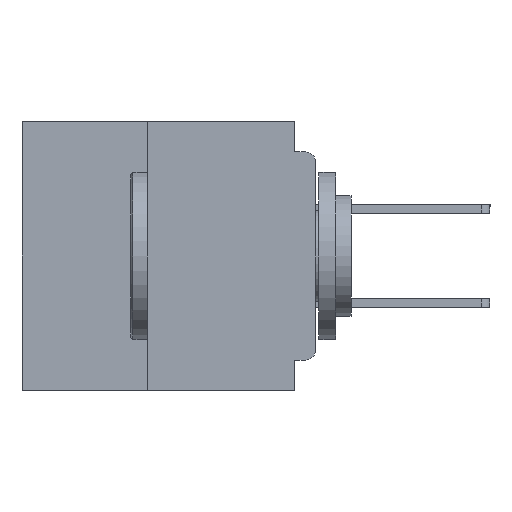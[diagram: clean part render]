
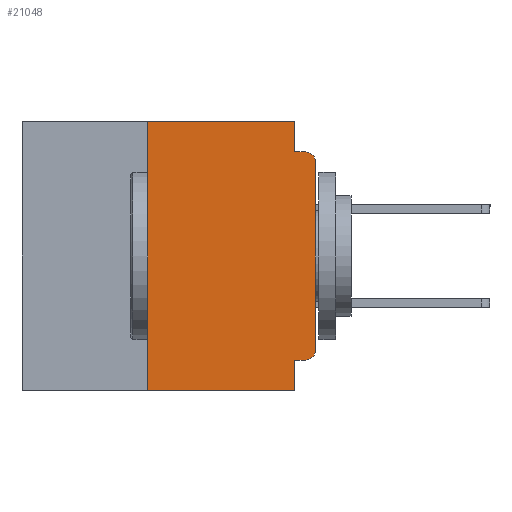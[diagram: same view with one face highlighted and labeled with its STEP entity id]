
A CAD part, left-side view. The second image highlights one B-rep face of the part: STEP entity #21048.
In plain terms, the highlighted planar face has unit normal (-1, 0, 0).
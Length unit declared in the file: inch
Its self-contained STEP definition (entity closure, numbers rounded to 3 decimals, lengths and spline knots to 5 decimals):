
#536 = CARTESIAN_POINT ( 'NONE',  ( 0., 0., -0.045 ) ) ;
#549 = DIRECTION ( 'NONE',  ( 0., -1., 0. ) ) ;
#659 = ORIENTED_EDGE ( 'NONE', *, *, #13368, .T. ) ;
#946 = CARTESIAN_POINT ( 'NONE',  ( 0., 0., -0.34 ) ) ;
#1817 = ORIENTED_EDGE ( 'NONE', *, *, #7299, .F. ) ;
#1946 = CARTESIAN_POINT ( 'NONE',  ( 0., 0.015, -0.34 ) ) ;
#2610 = DIRECTION ( 'NONE',  ( -1., 0., 0. ) ) ;
#2642 = EDGE_CURVE ( 'NONE', #10375, #23498, #8542, .T. ) ;
#2815 = ORIENTED_EDGE ( 'NONE', *, *, #8282, .F. ) ;
#3533 = ORIENTED_EDGE ( 'NONE', *, *, #5303, .F. ) ;
#4002 = VECTOR ( 'NONE', #20650, 39.37008 ) ;
#4003 = CARTESIAN_POINT ( 'NONE',  ( 0., 0.031, -0.355 ) ) ;
#4026 = EDGE_CURVE ( 'NONE', #25761, #7370, #26795, .T. ) ;
#4833 = LINE ( 'NONE', #11503, #26733 ) ;
#4872 = DIRECTION ( 'NONE',  ( 0., 0., -1. ) ) ;
#5227 = VERTEX_POINT ( 'NONE', #7113 ) ;
#5247 = DIRECTION ( 'NONE',  ( 0., 1., 0. ) ) ;
#5268 = CARTESIAN_POINT ( 'NONE',  ( 0., 0.25, -0.4 ) ) ;
#5276 = DIRECTION ( 'NONE',  ( 0., 0., 1. ) ) ;
#5303 = EDGE_CURVE ( 'NONE', #11004, #5783, #16511, .T. ) ;
#5427 = ORIENTED_EDGE ( 'NONE', *, *, #19109, .F. ) ;
#5503 = CARTESIAN_POINT ( 'NONE',  ( 0., 0.437, 0. ) ) ;
#5642 = ORIENTED_EDGE ( 'NONE', *, *, #19254, .F. ) ;
#5783 = VERTEX_POINT ( 'NONE', #35101 ) ;
#6601 = LINE ( 'NONE', #25414, #24919 ) ;
#7113 = CARTESIAN_POINT ( 'NONE',  ( 0., 0.031, -0.4 ) ) ;
#7151 = VECTOR ( 'NONE', #32325, 39.37008 ) ;
#7256 = ORIENTED_EDGE ( 'NONE', *, *, #33853, .T. ) ;
#7299 = EDGE_CURVE ( 'NONE', #7370, #25885, #13416, .T. ) ;
#7370 = VERTEX_POINT ( 'NONE', #14414 ) ;
#8282 = EDGE_CURVE ( 'NONE', #5783, #25761, #6601, .T. ) ;
#8411 = DIRECTION ( 'NONE',  ( 0., 0., -1. ) ) ;
#8455 = VECTOR ( 'NONE', #5247, 39.37008 ) ;
#8542 = LINE ( 'NONE', #18510, #36749 ) ;
#8766 = DIRECTION ( 'NONE',  ( 0., 0., -1. ) ) ;
#9298 = CARTESIAN_POINT ( 'NONE',  ( 0., 0.015, -0.045 ) ) ;
#10375 = VERTEX_POINT ( 'NONE', #946 ) ;
#11004 = VERTEX_POINT ( 'NONE', #28783 ) ;
#11503 = CARTESIAN_POINT ( 'NONE',  ( 0., 0.031, -0.4 ) ) ;
#12807 = CARTESIAN_POINT ( 'NONE',  ( 0., 0.015, -0.355 ) ) ;
#13368 = EDGE_CURVE ( 'NONE', #23498, #25885, #14032, .T. ) ;
#13416 = LINE ( 'NONE', #536, #27639 ) ;
#13871 = CIRCLE ( 'NONE', #25834, 0.015 ) ;
#14007 = VERTEX_POINT ( 'NONE', #12807 ) ;
#14032 = CIRCLE ( 'NONE', #20231, 0.015 ) ;
#14414 = CARTESIAN_POINT ( 'NONE',  ( 0., 0.031, -0.045 ) ) ;
#15114 = CARTESIAN_POINT ( 'NONE',  ( 0., 0.437, -0.4 ) ) ;
#16034 = CARTESIAN_POINT ( 'NONE',  ( 0., 0., -0.06 ) ) ;
#16511 = LINE ( 'NONE', #5268, #22205 ) ;
#16725 = CARTESIAN_POINT ( 'NONE',  ( 0., 0., -0.355 ) ) ;
#18510 = CARTESIAN_POINT ( 'NONE',  ( 0., 0., 0. ) ) ;
#18836 = DIRECTION ( 'NONE',  ( 0., 0., 1. ) ) ;
#19017 = EDGE_CURVE ( 'NONE', #14007, #10375, #13871, .T. ) ;
#19109 = EDGE_CURVE ( 'NONE', #14007, #28911, #31119, .T. ) ;
#19254 = EDGE_CURVE ( 'NONE', #28911, #5227, #4833, .T. ) ;
#19842 = CARTESIAN_POINT ( 'NONE',  ( 0., 0.015, -0.06 ) ) ;
#20231 = AXIS2_PLACEMENT_3D ( 'NONE', #19842, #2610, #22641 ) ;
#20279 = EDGE_LOOP ( 'NONE', ( #28506, #659, #1817, #29278, #2815, #3533, #7256, #5642, #5427, #32223 ) ) ;
#20650 = DIRECTION ( 'NONE',  ( 0., -1., 0. ) ) ;
#21048 = ADVANCED_FACE ( 'NONE', ( #29656 ), #31014, .F. ) ;
#21980 = DIRECTION ( 'NONE',  ( -1., 0., 0. ) ) ;
#22205 = VECTOR ( 'NONE', #5276, 39.37008 ) ;
#22641 = DIRECTION ( 'NONE',  ( 0., 0., -1. ) ) ;
#22741 = AXIS2_PLACEMENT_3D ( 'NONE', #5503, #25501, #8411 ) ;
#23498 = VERTEX_POINT ( 'NONE', #16034 ) ;
#24919 = VECTOR ( 'NONE', #31051, 39.37008 ) ;
#25414 = CARTESIAN_POINT ( 'NONE',  ( 0., 0.437, 0. ) ) ;
#25501 = DIRECTION ( 'NONE',  ( 1., 0., 0. ) ) ;
#25742 = CARTESIAN_POINT ( 'NONE',  ( 0., 0.031, 0. ) ) ;
#25761 = VERTEX_POINT ( 'NONE', #25742 ) ;
#25834 = AXIS2_PLACEMENT_3D ( 'NONE', #1946, #21980, #4872 ) ;
#25885 = VERTEX_POINT ( 'NONE', #9298 ) ;
#25927 = LINE ( 'NONE', #15114, #4002 ) ;
#26733 = VECTOR ( 'NONE', #8766, 39.37008 ) ;
#26795 = LINE ( 'NONE', #32157, #7151 ) ;
#27639 = VECTOR ( 'NONE', #549, 39.37008 ) ;
#28506 = ORIENTED_EDGE ( 'NONE', *, *, #2642, .T. ) ;
#28783 = CARTESIAN_POINT ( 'NONE',  ( 0., 0.25, -0.4 ) ) ;
#28911 = VERTEX_POINT ( 'NONE', #4003 ) ;
#29278 = ORIENTED_EDGE ( 'NONE', *, *, #4026, .F. ) ;
#29656 = FACE_OUTER_BOUND ( 'NONE', #20279, .T. ) ;
#31014 = PLANE ( 'NONE',  #22741 ) ;
#31051 = DIRECTION ( 'NONE',  ( 0., -1., 0. ) ) ;
#31119 = LINE ( 'NONE', #16725, #8455 ) ;
#32157 = CARTESIAN_POINT ( 'NONE',  ( 0., 0.031, 0. ) ) ;
#32223 = ORIENTED_EDGE ( 'NONE', *, *, #19017, .T. ) ;
#32325 = DIRECTION ( 'NONE',  ( 0., 0., -1. ) ) ;
#33853 = EDGE_CURVE ( 'NONE', #11004, #5227, #25927, .T. ) ;
#35101 = CARTESIAN_POINT ( 'NONE',  ( 0., 0.25, 0. ) ) ;
#36749 = VECTOR ( 'NONE', #18836, 39.37008 ) ;
